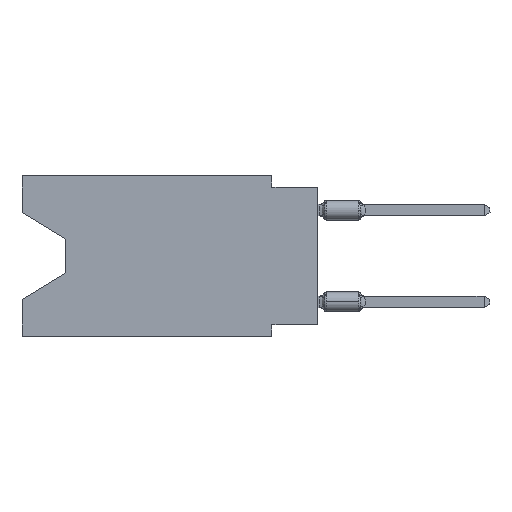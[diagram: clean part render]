
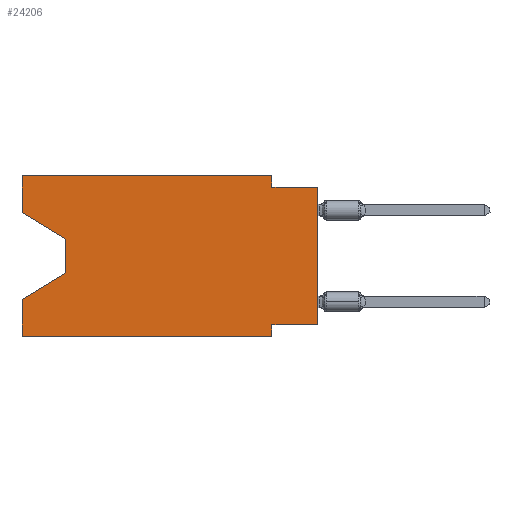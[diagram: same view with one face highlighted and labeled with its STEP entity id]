
A CAD part, left-side view. The second image highlights one B-rep face of the part: STEP entity #24206.
In plain terms, the highlighted planar face has unit normal (-1, 0, 0).
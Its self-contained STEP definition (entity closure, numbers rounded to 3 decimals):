
#63 = ORIENTED_EDGE ( 'NONE', *, *, #12163, .F. ) ;
#110 = EDGE_CURVE ( 'NONE', #4242, #20784, #15021, .T. ) ;
#145 = VERTEX_POINT ( 'NONE', #22440 ) ;
#701 = LINE ( 'NONE', #5092, #11464 ) ;
#849 = DIRECTION ( 'NONE',  ( 0., 0., -1. ) ) ;
#1726 = ORIENTED_EDGE ( 'NONE', *, *, #17139, .F. ) ;
#2174 = DIRECTION ( 'NONE',  ( 0., -1., 0. ) ) ;
#2286 = VECTOR ( 'NONE', #12765, 1000. ) ;
#2455 = VERTEX_POINT ( 'NONE', #19129 ) ;
#2581 = ORIENTED_EDGE ( 'NONE', *, *, #12914, .F. ) ;
#2761 = DIRECTION ( 'NONE',  ( 0., 0.855, -0.519 ) ) ;
#2766 = ORIENTED_EDGE ( 'NONE', *, *, #25310, .F. ) ;
#2929 = EDGE_CURVE ( 'NONE', #4255, #21670, #27633, .T. ) ;
#2967 = DIRECTION ( 'NONE',  ( 0., 0., 1. ) ) ;
#3028 = DIRECTION ( 'NONE',  ( 1., 0., 0. ) ) ;
#3154 = ORIENTED_EDGE ( 'NONE', *, *, #2929, .T. ) ;
#3431 = DIRECTION ( 'NONE',  ( 0., 0., 1. ) ) ;
#3749 = DIRECTION ( 'NONE',  ( 0., -1., 0. ) ) ;
#4173 = CARTESIAN_POINT ( 'NONE',  ( 0., 0., -8.255 ) ) ;
#4242 = VERTEX_POINT ( 'NONE', #27217 ) ;
#4255 = VERTEX_POINT ( 'NONE', #7940 ) ;
#4667 = LINE ( 'NONE', #6843, #15744 ) ;
#5089 = PLANE ( 'NONE',  #6847 ) ;
#5092 = CARTESIAN_POINT ( 'NONE',  ( 0., 13.97, -5.385 ) ) ;
#5282 = EDGE_LOOP ( 'NONE', ( #3154, #17587, #8182, #63, #8041, #2581, #2766, #13325, #26679, #1726, #6738, #15388 ) ) ;
#5836 = EDGE_CURVE ( 'NONE', #4255, #4242, #26308, .T. ) ;
#5970 = VECTOR ( 'NONE', #8601, 1000. ) ;
#6628 = CARTESIAN_POINT ( 'NONE',  ( 0., 2.54, 0. ) ) ;
#6738 = ORIENTED_EDGE ( 'NONE', *, *, #110, .F. ) ;
#6843 = CARTESIAN_POINT ( 'NONE',  ( 0., 16.383, -8.89 ) ) ;
#6847 = AXIS2_PLACEMENT_3D ( 'NONE', #13720, #3028, #849 ) ;
#7482 = VERTEX_POINT ( 'NONE', #20633 ) ;
#7940 = CARTESIAN_POINT ( 'NONE',  ( 0., 16.383, -2.038 ) ) ;
#7946 = VECTOR ( 'NONE', #27133, 1000. ) ;
#7950 = VECTOR ( 'NONE', #3749, 1000. ) ;
#8041 = ORIENTED_EDGE ( 'NONE', *, *, #15244, .T. ) ;
#8182 = ORIENTED_EDGE ( 'NONE', *, *, #22744, .T. ) ;
#8382 = LINE ( 'NONE', #25988, #16746 ) ;
#8385 = LINE ( 'NONE', #9104, #10694 ) ;
#8523 = CARTESIAN_POINT ( 'NONE',  ( 0., 16.383, -2.038 ) ) ;
#8601 = DIRECTION ( 'NONE',  ( 0., 1., 0. ) ) ;
#9104 = CARTESIAN_POINT ( 'NONE',  ( 0., 0., 0. ) ) ;
#9221 = LINE ( 'NONE', #18175, #7946 ) ;
#10438 = DIRECTION ( 'NONE',  ( 0., 0., -1. ) ) ;
#10694 = VECTOR ( 'NONE', #2967, 1000. ) ;
#10977 = VERTEX_POINT ( 'NONE', #16268 ) ;
#11464 = VECTOR ( 'NONE', #2761, 1000. ) ;
#12080 = VECTOR ( 'NONE', #10438, 1000. ) ;
#12163 = EDGE_CURVE ( 'NONE', #10977, #145, #8382, .T. ) ;
#12490 = CARTESIAN_POINT ( 'NONE',  ( 0., 2.54, -8.255 ) ) ;
#12765 = DIRECTION ( 'NONE',  ( 0., -0.855, -0.519 ) ) ;
#12914 = EDGE_CURVE ( 'NONE', #25857, #7482, #9221, .T. ) ;
#13275 = LINE ( 'NONE', #22218, #27461 ) ;
#13325 = ORIENTED_EDGE ( 'NONE', *, *, #26149, .T. ) ;
#13379 = VECTOR ( 'NONE', #21947, 1000. ) ;
#13720 = CARTESIAN_POINT ( 'NONE',  ( 0., 16.383, 0. ) ) ;
#15021 = LINE ( 'NONE', #17508, #7950 ) ;
#15244 = EDGE_CURVE ( 'NONE', #10977, #7482, #4667, .T. ) ;
#15388 = ORIENTED_EDGE ( 'NONE', *, *, #5836, .F. ) ;
#15513 = CARTESIAN_POINT ( 'NONE',  ( 0., 0., -8.255 ) ) ;
#15744 = VECTOR ( 'NONE', #2174, 1000. ) ;
#16268 = CARTESIAN_POINT ( 'NONE',  ( 0., 16.383, -8.89 ) ) ;
#16746 = VECTOR ( 'NONE', #3431, 1000. ) ;
#17139 = EDGE_CURVE ( 'NONE', #20784, #24672, #23947, .T. ) ;
#17508 = CARTESIAN_POINT ( 'NONE',  ( 0., 16.383, 0. ) ) ;
#17574 = VERTEX_POINT ( 'NONE', #19661 ) ;
#17587 = ORIENTED_EDGE ( 'NONE', *, *, #24113, .T. ) ;
#18143 = LINE ( 'NONE', #15513, #5970 ) ;
#18175 = CARTESIAN_POINT ( 'NONE',  ( 0., 2.54, -8.89 ) ) ;
#18240 = VECTOR ( 'NONE', #26449, 1000. ) ;
#18259 = CARTESIAN_POINT ( 'NONE',  ( 0., 13.97, -3.505 ) ) ;
#18379 = CARTESIAN_POINT ( 'NONE',  ( 0., 2.54, -0.635 ) ) ;
#18412 = FACE_OUTER_BOUND ( 'NONE', #5282, .T. ) ;
#19129 = CARTESIAN_POINT ( 'NONE',  ( 0., 13.97, -5.385 ) ) ;
#19661 = CARTESIAN_POINT ( 'NONE',  ( 0., 0., -0.635 ) ) ;
#20633 = CARTESIAN_POINT ( 'NONE',  ( 0., 2.54, -8.89 ) ) ;
#20784 = VERTEX_POINT ( 'NONE', #6628 ) ;
#21670 = VERTEX_POINT ( 'NONE', #18259 ) ;
#21947 = DIRECTION ( 'NONE',  ( 0., -1., 0. ) ) ;
#22218 = CARTESIAN_POINT ( 'NONE',  ( 0., 13.97, -3.505 ) ) ;
#22316 = CARTESIAN_POINT ( 'NONE',  ( 0., 16.383, 0. ) ) ;
#22369 = LINE ( 'NONE', #26660, #13379 ) ;
#22440 = CARTESIAN_POINT ( 'NONE',  ( 0., 16.383, -6.852 ) ) ;
#22744 = EDGE_CURVE ( 'NONE', #2455, #145, #701, .T. ) ;
#23947 = LINE ( 'NONE', #28641, #12080 ) ;
#24041 = EDGE_CURVE ( 'NONE', #24672, #17574, #22369, .T. ) ;
#24113 = EDGE_CURVE ( 'NONE', #21670, #2455, #13275, .T. ) ;
#24206 = ADVANCED_FACE ( 'NONE', ( #18412 ), #5089, .F. ) ;
#24573 = DIRECTION ( 'NONE',  ( 0., 0., -1. ) ) ;
#24672 = VERTEX_POINT ( 'NONE', #18379 ) ;
#25310 = EDGE_CURVE ( 'NONE', #26843, #25857, #18143, .T. ) ;
#25857 = VERTEX_POINT ( 'NONE', #12490 ) ;
#25988 = CARTESIAN_POINT ( 'NONE',  ( 0., 16.383, 0. ) ) ;
#26149 = EDGE_CURVE ( 'NONE', #26843, #17574, #8385, .T. ) ;
#26308 = LINE ( 'NONE', #22316, #18240 ) ;
#26449 = DIRECTION ( 'NONE',  ( 0., 0., 1. ) ) ;
#26660 = CARTESIAN_POINT ( 'NONE',  ( 0., 0., -0.635 ) ) ;
#26679 = ORIENTED_EDGE ( 'NONE', *, *, #24041, .F. ) ;
#26843 = VERTEX_POINT ( 'NONE', #4173 ) ;
#27133 = DIRECTION ( 'NONE',  ( 0., 0., -1. ) ) ;
#27217 = CARTESIAN_POINT ( 'NONE',  ( 0., 16.383, 0. ) ) ;
#27461 = VECTOR ( 'NONE', #24573, 1000. ) ;
#27633 = LINE ( 'NONE', #8523, #2286 ) ;
#28641 = CARTESIAN_POINT ( 'NONE',  ( 0., 2.54, 0. ) ) ;
